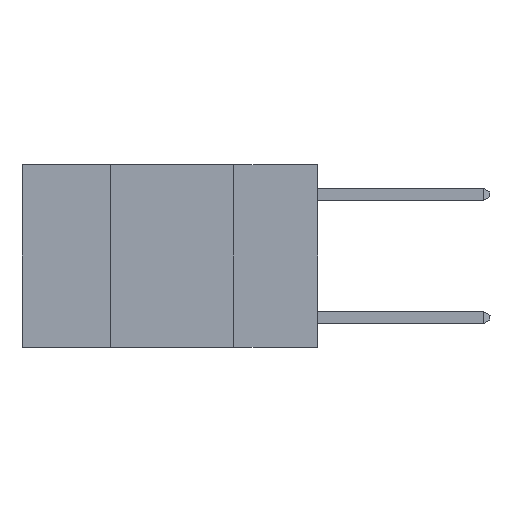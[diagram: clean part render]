
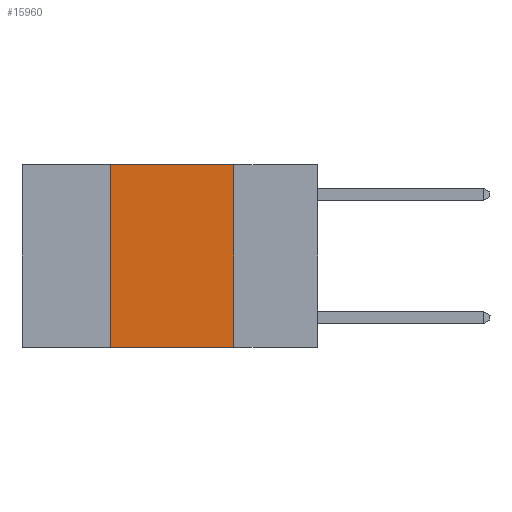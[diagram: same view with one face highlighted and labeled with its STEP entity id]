
A CAD part, left-side view. The second image highlights one B-rep face of the part: STEP entity #15960.
In plain terms, the highlighted planar face has unit normal (-1, 0, 0).
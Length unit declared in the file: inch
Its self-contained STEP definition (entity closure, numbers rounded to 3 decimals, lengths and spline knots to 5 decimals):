
#1234 = VERTEX_POINT ( 'NONE', #19896 ) ;
#1492 = ORIENTED_EDGE ( 'NONE', *, *, #9945, .F. ) ;
#2124 = CARTESIAN_POINT ( 'NONE',  ( 0., 0.42, 0. ) ) ;
#3619 = DIRECTION ( 'NONE',  ( 0., 0., -1. ) ) ;
#3995 = EDGE_LOOP ( 'NONE', ( #1492, #6218, #7308, #12002 ) ) ;
#5013 = DIRECTION ( 'NONE',  ( 0., -1., 0. ) ) ;
#5090 = CARTESIAN_POINT ( 'NONE',  ( 0., 0.6, 0. ) ) ;
#6218 = ORIENTED_EDGE ( 'NONE', *, *, #21409, .F. ) ;
#6846 = CARTESIAN_POINT ( 'NONE',  ( 0., 0.42, 0. ) ) ;
#7118 = LINE ( 'NONE', #22835, #11812 ) ;
#7308 = ORIENTED_EDGE ( 'NONE', *, *, #12339, .F. ) ;
#7890 = DIRECTION ( 'NONE',  ( 1., 0., 0. ) ) ;
#8400 = LINE ( 'NONE', #2124, #22578 ) ;
#9527 = VERTEX_POINT ( 'NONE', #19875 ) ;
#9563 = VECTOR ( 'NONE', #5013, 39.37008 ) ;
#9945 = EDGE_CURVE ( 'NONE', #1234, #9527, #20368, .T. ) ;
#10883 = VECTOR ( 'NONE', #3619, 39.37008 ) ;
#11360 = AXIS2_PLACEMENT_3D ( 'NONE', #14973, #7890, #20313 ) ;
#11812 = VECTOR ( 'NONE', #12206, 39.37008 ) ;
#12002 = ORIENTED_EDGE ( 'NONE', *, *, #20957, .T. ) ;
#12206 = DIRECTION ( 'NONE',  ( 0., -1., 0. ) ) ;
#12339 = EDGE_CURVE ( 'NONE', #18189, #16776, #8400, .T. ) ;
#14337 = LINE ( 'NONE', #5090, #9563 ) ;
#14555 = DIRECTION ( 'NONE',  ( 0., 0., 1. ) ) ;
#14973 = CARTESIAN_POINT ( 'NONE',  ( 0., 0.6, 0. ) ) ;
#15960 = ADVANCED_FACE ( 'NONE', ( #20511 ), #18520, .F. ) ;
#16776 = VERTEX_POINT ( 'NONE', #6846 ) ;
#18189 = VERTEX_POINT ( 'NONE', #19667 ) ;
#18520 = PLANE ( 'NONE',  #11360 ) ;
#19591 = CARTESIAN_POINT ( 'NONE',  ( 0., 0.17, 0. ) ) ;
#19667 = CARTESIAN_POINT ( 'NONE',  ( 0., 0.42, -0.37 ) ) ;
#19875 = CARTESIAN_POINT ( 'NONE',  ( 0., 0.17, -0.37 ) ) ;
#19896 = CARTESIAN_POINT ( 'NONE',  ( 0., 0.17, 0. ) ) ;
#20313 = DIRECTION ( 'NONE',  ( 0., 0., -1. ) ) ;
#20368 = LINE ( 'NONE', #19591, #10883 ) ;
#20511 = FACE_OUTER_BOUND ( 'NONE', #3995, .T. ) ;
#20957 = EDGE_CURVE ( 'NONE', #18189, #9527, #7118, .T. ) ;
#21409 = EDGE_CURVE ( 'NONE', #16776, #1234, #14337, .T. ) ;
#22578 = VECTOR ( 'NONE', #14555, 39.37008 ) ;
#22835 = CARTESIAN_POINT ( 'NONE',  ( 0., 0.6, -0.37 ) ) ;
